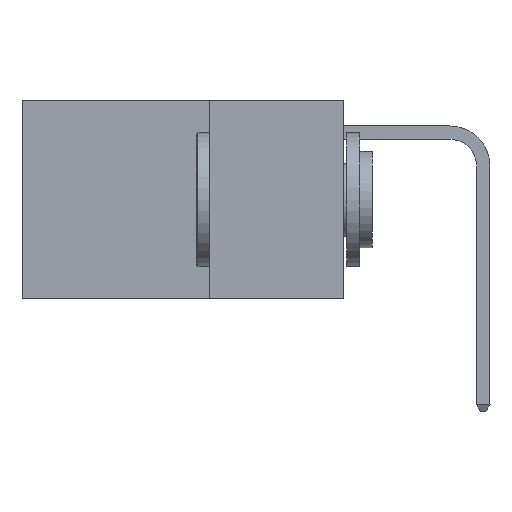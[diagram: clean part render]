
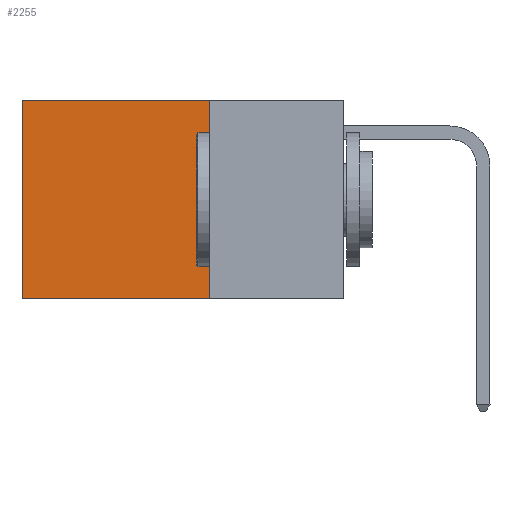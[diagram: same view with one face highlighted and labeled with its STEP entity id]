
A CAD part, left-side view. The second image highlights one B-rep face of the part: STEP entity #2255.
In plain terms, the highlighted planar face has unit normal (-1, 0, 0).
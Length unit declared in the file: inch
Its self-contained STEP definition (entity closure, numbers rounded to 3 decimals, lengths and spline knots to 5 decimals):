
#86 = LINE ( 'NONE', #5671, #1396 ) ;
#88 = EDGE_CURVE ( 'NONE', #10911, #1399, #9626, .T. ) ;
#300 = DIRECTION ( 'NONE',  ( 0., 0., -1. ) ) ;
#428 = FACE_OUTER_BOUND ( 'NONE', #1031, .T. ) ;
#657 = LINE ( 'NONE', #8176, #1957 ) ;
#1031 = EDGE_LOOP ( 'NONE', ( #11010, #10377, #4967, #1984 ) ) ;
#1209 = CARTESIAN_POINT ( 'NONE',  ( 0.2625, 0.25, 0. ) ) ;
#1396 = VECTOR ( 'NONE', #3834, 39.37008 ) ;
#1399 = VERTEX_POINT ( 'NONE', #6112 ) ;
#1957 = VECTOR ( 'NONE', #5366, 39.37008 ) ;
#1984 = ORIENTED_EDGE ( 'NONE', *, *, #4239, .T. ) ;
#2191 = DIRECTION ( 'NONE',  ( 1., 0., 0. ) ) ;
#2255 = ADVANCED_FACE ( 'NONE', ( #428 ), #8743, .F. ) ;
#2384 = CARTESIAN_POINT ( 'NONE',  ( 0.2625, 0.6, 0. ) ) ;
#2467 = VERTEX_POINT ( 'NONE', #2564 ) ;
#2564 = CARTESIAN_POINT ( 'NONE',  ( 0.2625, 0.6, 0. ) ) ;
#2691 = VECTOR ( 'NONE', #7213, 39.37008 ) ;
#3537 = VERTEX_POINT ( 'NONE', #11946 ) ;
#3594 = CARTESIAN_POINT ( 'NONE',  ( 0.2625, 0.25, 0. ) ) ;
#3749 = VECTOR ( 'NONE', #11700, 39.37008 ) ;
#3834 = DIRECTION ( 'NONE',  ( 0., 1., 0. ) ) ;
#4222 = EDGE_CURVE ( 'NONE', #1399, #3537, #657, .T. ) ;
#4239 = EDGE_CURVE ( 'NONE', #10911, #2467, #86, .T. ) ;
#4967 = ORIENTED_EDGE ( 'NONE', *, *, #88, .F. ) ;
#5011 = EDGE_CURVE ( 'NONE', #2467, #3537, #8993, .T. ) ;
#5366 = DIRECTION ( 'NONE',  ( 0., 1., 0. ) ) ;
#5671 = CARTESIAN_POINT ( 'NONE',  ( 0.2625, 0.25, 0. ) ) ;
#6112 = CARTESIAN_POINT ( 'NONE',  ( 0.2625, 0.25, -0.37 ) ) ;
#7213 = DIRECTION ( 'NONE',  ( 0., 0., -1. ) ) ;
#8176 = CARTESIAN_POINT ( 'NONE',  ( 0.2625, 0.25, -0.37 ) ) ;
#8743 = PLANE ( 'NONE',  #11792 ) ;
#8993 = LINE ( 'NONE', #2384, #3749 ) ;
#9626 = LINE ( 'NONE', #1209, #2691 ) ;
#9825 = CARTESIAN_POINT ( 'NONE',  ( 0.2625, 0.25, 0. ) ) ;
#10377 = ORIENTED_EDGE ( 'NONE', *, *, #4222, .F. ) ;
#10911 = VERTEX_POINT ( 'NONE', #3594 ) ;
#11010 = ORIENTED_EDGE ( 'NONE', *, *, #5011, .T. ) ;
#11700 = DIRECTION ( 'NONE',  ( 0., 0., -1. ) ) ;
#11792 = AXIS2_PLACEMENT_3D ( 'NONE', #9825, #2191, #300 ) ;
#11946 = CARTESIAN_POINT ( 'NONE',  ( 0.2625, 0.6, -0.37 ) ) ;
